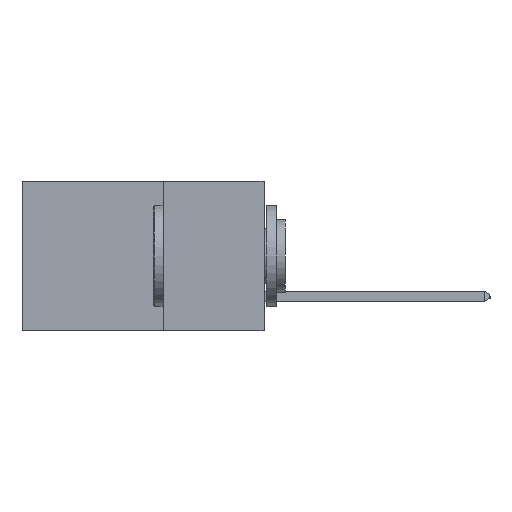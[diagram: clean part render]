
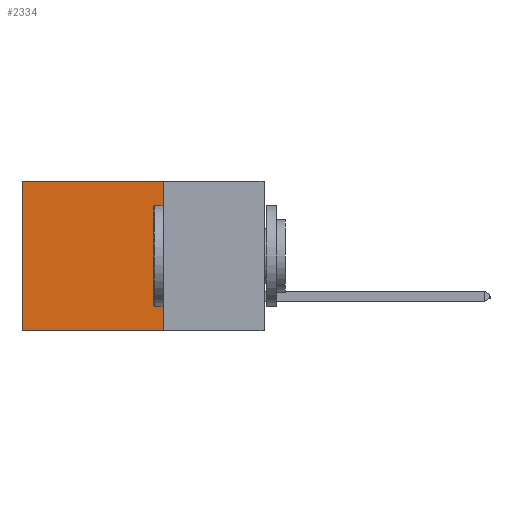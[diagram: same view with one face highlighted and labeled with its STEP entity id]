
A CAD part, left-side view. The second image highlights one B-rep face of the part: STEP entity #2334.
In plain terms, the highlighted planar face has unit normal (-1, 0, 0).
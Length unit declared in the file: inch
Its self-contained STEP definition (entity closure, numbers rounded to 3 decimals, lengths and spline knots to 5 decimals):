
#226 = VECTOR ( 'NONE', #7169, 39.37008 ) ;
#871 = DIRECTION ( 'NONE',  ( 0., 0., -1. ) ) ;
#895 = ORIENTED_EDGE ( 'NONE', *, *, #14534, .T. ) ;
#1834 = VERTEX_POINT ( 'NONE', #15317 ) ;
#1908 = CARTESIAN_POINT ( 'NONE',  ( 0.298, 0.6, 0. ) ) ;
#2023 = VECTOR ( 'NONE', #7226, 39.37008 ) ;
#2334 = ADVANCED_FACE ( 'NONE', ( #9031 ), #6904, .F. ) ;
#2795 = LINE ( 'NONE', #12799, #15208 ) ;
#3452 = CARTESIAN_POINT ( 'NONE',  ( 0.298, 0.25, 0. ) ) ;
#4654 = CARTESIAN_POINT ( 'NONE',  ( 0.298, 0.6, 0. ) ) ;
#5330 = ORIENTED_EDGE ( 'NONE', *, *, #10702, .F. ) ;
#6153 = DIRECTION ( 'NONE',  ( 0., 0., -1. ) ) ;
#6904 = PLANE ( 'NONE',  #10432 ) ;
#7169 = DIRECTION ( 'NONE',  ( 0., 1., 0. ) ) ;
#7226 = DIRECTION ( 'NONE',  ( 0., 0., -1. ) ) ;
#7465 = CARTESIAN_POINT ( 'NONE',  ( 0.298, 0.25, 0. ) ) ;
#7547 = DIRECTION ( 'NONE',  ( 0., 1., 0. ) ) ;
#7757 = DIRECTION ( 'NONE',  ( 1., 0., 0. ) ) ;
#9031 = FACE_OUTER_BOUND ( 'NONE', #13853, .T. ) ;
#9149 = EDGE_CURVE ( 'NONE', #14825, #1834, #14463, .T. ) ;
#9205 = VERTEX_POINT ( 'NONE', #1908 ) ;
#9404 = LINE ( 'NONE', #3452, #15992 ) ;
#9518 = LINE ( 'NONE', #4654, #2023 ) ;
#10432 = AXIS2_PLACEMENT_3D ( 'NONE', #14658, #7757, #871 ) ;
#10702 = EDGE_CURVE ( 'NONE', #13420, #14825, #9404, .T. ) ;
#10752 = EDGE_CURVE ( 'NONE', #13420, #9205, #2795, .T. ) ;
#12799 = CARTESIAN_POINT ( 'NONE',  ( 0.298, 0.25, 0. ) ) ;
#12878 = ORIENTED_EDGE ( 'NONE', *, *, #10752, .T. ) ;
#13420 = VERTEX_POINT ( 'NONE', #7465 ) ;
#13748 = CARTESIAN_POINT ( 'NONE',  ( 0.298, 0.25, -0.37 ) ) ;
#13853 = EDGE_LOOP ( 'NONE', ( #895, #15151, #5330, #12878 ) ) ;
#14463 = LINE ( 'NONE', #13748, #226 ) ;
#14478 = CARTESIAN_POINT ( 'NONE',  ( 0.298, 0.25, -0.37 ) ) ;
#14534 = EDGE_CURVE ( 'NONE', #9205, #1834, #9518, .T. ) ;
#14658 = CARTESIAN_POINT ( 'NONE',  ( 0.298, 0.25, 0. ) ) ;
#14825 = VERTEX_POINT ( 'NONE', #14478 ) ;
#15151 = ORIENTED_EDGE ( 'NONE', *, *, #9149, .F. ) ;
#15208 = VECTOR ( 'NONE', #7547, 39.37008 ) ;
#15317 = CARTESIAN_POINT ( 'NONE',  ( 0.298, 0.6, -0.37 ) ) ;
#15992 = VECTOR ( 'NONE', #6153, 39.37008 ) ;
